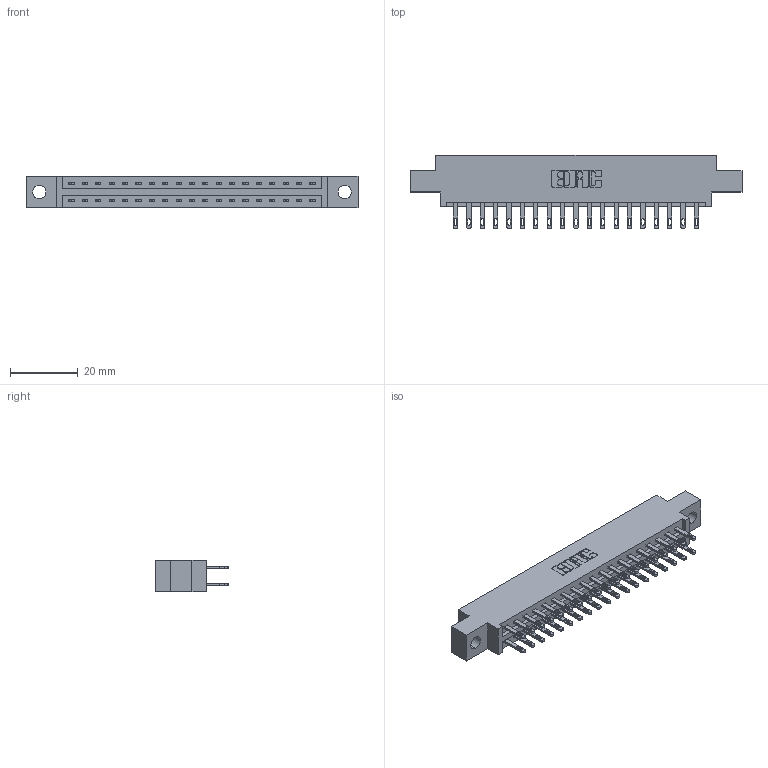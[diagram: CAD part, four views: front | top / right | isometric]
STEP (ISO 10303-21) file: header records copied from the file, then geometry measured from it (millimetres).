
FILE_DESCRIPTION (( 'STEP AP203' ), '1' );
FILE_NAME ('887-038-500-804.STEP', '2020-09-20T22:58:36', ( '' ), ( '' ), 'SwSTEP 2.0', 'SolidWorks 2020', '' );
FILE_SCHEMA (( 'CONFIG_CONTROL_DESIGN' ));
Length unit declared in the file: inch
Products named in the file (3): 345-292-001_345-293-100; 837 Part_0.170 Offset - 0.156 Dia-TH; 887-038-500-804
Assembly tree (39 placements, depth 2):
  887-038-500-804
    837 Part_0.170 Offset - 0.156 Dia-TH
    345-292-001_345-293-100  x38
Bounding box: 98.3 x 21.85 x 9.4 mm (x, y, z)
Volume: 9964 mm3; surface area: 11367.8 mm2
Topology: 39 solids, 39 shells, 2018 faces, 6137 edges, 4090 vertices
Faces by surface type: plane 1290, cylinder 728
Entity records: 17771 total; most frequent: CARTESIAN_POINT 3014, ORIENTED_EDGE 2950, DIRECTION 2607, EDGE_CURVE 1475, LINE 1343, VECTOR 1343, VERTEX_POINT 982, AXIS2_PLACEMENT_3D 632
